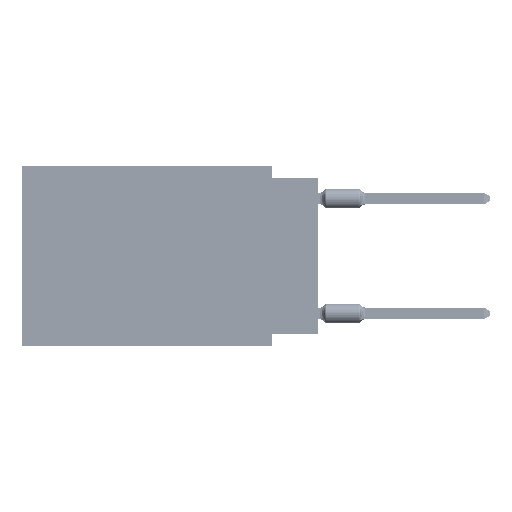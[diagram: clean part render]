
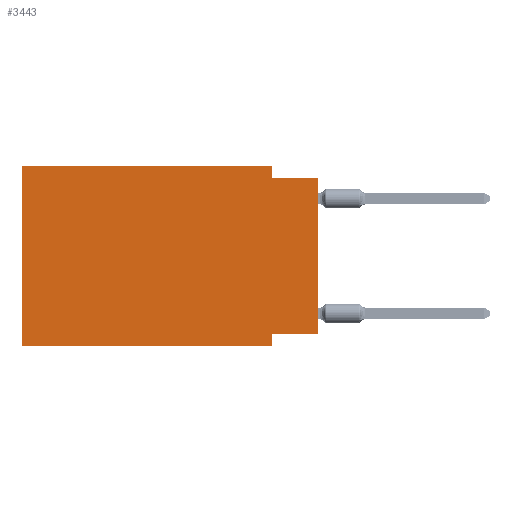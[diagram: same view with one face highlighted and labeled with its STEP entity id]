
A CAD part, left-side view. The second image highlights one B-rep face of the part: STEP entity #3443.
In plain terms, the highlighted planar face has unit normal (-1, 0, 0).
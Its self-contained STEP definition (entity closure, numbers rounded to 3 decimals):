
#3443 = ADVANCED_FACE ( 'NONE', ( #73398 ), #48200, .F. ) ;
#3777 = CARTESIAN_POINT ( 'NONE',  ( 0., 16.383, -9.906 ) ) ;
#6930 = VECTOR ( 'NONE', #9589, 1000. ) ;
#7085 = LINE ( 'NONE', #56255, #73986 ) ;
#7325 = LINE ( 'NONE', #38696, #23880 ) ;
#7594 = EDGE_CURVE ( 'NONE', #34533, #52376, #45774, .T. ) ;
#8217 = VERTEX_POINT ( 'NONE', #70680 ) ;
#9589 = DIRECTION ( 'NONE',  ( 0., -1., 0. ) ) ;
#9990 = LINE ( 'NONE', #3777, #6930 ) ;
#12648 = EDGE_LOOP ( 'NONE', ( #13565, #73922, #52273, #21023, #25241, #41100, #47008, #46604 ) ) ;
#13565 = ORIENTED_EDGE ( 'NONE', *, *, #61084, .T. ) ;
#16958 = EDGE_CURVE ( 'NONE', #50611, #20194, #9990, .T. ) ;
#19933 = DIRECTION ( 'NONE',  ( 0., 0., -1. ) ) ;
#20194 = VERTEX_POINT ( 'NONE', #63922 ) ;
#21023 = ORIENTED_EDGE ( 'NONE', *, *, #24905, .F. ) ;
#21789 = DIRECTION ( 'NONE',  ( 0., -1., 0. ) ) ;
#23021 = DIRECTION ( 'NONE',  ( 0., 0., -1. ) ) ;
#23880 = VECTOR ( 'NONE', #32113, 1000. ) ;
#24905 = EDGE_CURVE ( 'NONE', #73498, #34533, #7085, .T. ) ;
#25241 = ORIENTED_EDGE ( 'NONE', *, *, #78553, .F. ) ;
#26257 = VECTOR ( 'NONE', #19933, 1000. ) ;
#26548 = CARTESIAN_POINT ( 'NONE',  ( 0., 2.54, -9.906 ) ) ;
#28458 = CARTESIAN_POINT ( 'NONE',  ( 0., 16.383, 0. ) ) ;
#29220 = DIRECTION ( 'NONE',  ( 1., 0., 0. ) ) ;
#29319 = CARTESIAN_POINT ( 'NONE',  ( 0., 2.54, -9.271 ) ) ;
#29697 = CARTESIAN_POINT ( 'NONE',  ( 0., 2.54, -0.635 ) ) ;
#29850 = DIRECTION ( 'NONE',  ( 0., 1., 0. ) ) ;
#32113 = DIRECTION ( 'NONE',  ( 0., 0., 1. ) ) ;
#34517 = EDGE_CURVE ( 'NONE', #54607, #51164, #46826, .T. ) ;
#34533 = VERTEX_POINT ( 'NONE', #59631 ) ;
#36315 = VECTOR ( 'NONE', #80869, 1000. ) ;
#36653 = LINE ( 'NONE', #68861, #36315 ) ;
#37709 = LINE ( 'NONE', #26548, #26257 ) ;
#38696 = CARTESIAN_POINT ( 'NONE',  ( 0., 0., 0. ) ) ;
#39715 = AXIS2_PLACEMENT_3D ( 'NONE', #41190, #29220, #23021 ) ;
#41100 = ORIENTED_EDGE ( 'NONE', *, *, #16958, .T. ) ;
#41190 = CARTESIAN_POINT ( 'NONE',  ( 0., 16.383, 0. ) ) ;
#45774 = LINE ( 'NONE', #53606, #58546 ) ;
#46604 = ORIENTED_EDGE ( 'NONE', *, *, #34517, .F. ) ;
#46661 = CARTESIAN_POINT ( 'NONE',  ( 0., 0., -9.271 ) ) ;
#46826 = LINE ( 'NONE', #72015, #73651 ) ;
#47008 = ORIENTED_EDGE ( 'NONE', *, *, #67444, .F. ) ;
#48200 = PLANE ( 'NONE',  #39715 ) ;
#50611 = VERTEX_POINT ( 'NONE', #63854 ) ;
#50863 = DIRECTION ( 'NONE',  ( 0., -1., 0. ) ) ;
#51164 = VERTEX_POINT ( 'NONE', #29319 ) ;
#52273 = ORIENTED_EDGE ( 'NONE', *, *, #7594, .F. ) ;
#52376 = VERTEX_POINT ( 'NONE', #29697 ) ;
#53606 = CARTESIAN_POINT ( 'NONE',  ( 0., 2.54, 0. ) ) ;
#54607 = VERTEX_POINT ( 'NONE', #46661 ) ;
#56255 = CARTESIAN_POINT ( 'NONE',  ( 0., 16.383, 0. ) ) ;
#58546 = VECTOR ( 'NONE', #78404, 1000. ) ;
#58986 = CARTESIAN_POINT ( 'NONE',  ( 0., 0., -0.635 ) ) ;
#59631 = CARTESIAN_POINT ( 'NONE',  ( 0., 2.54, 0. ) ) ;
#61084 = EDGE_CURVE ( 'NONE', #54607, #8217, #7325, .T. ) ;
#63854 = CARTESIAN_POINT ( 'NONE',  ( 0., 16.383, -9.906 ) ) ;
#63922 = CARTESIAN_POINT ( 'NONE',  ( 0., 2.54, -9.906 ) ) ;
#67444 = EDGE_CURVE ( 'NONE', #51164, #20194, #37709, .T. ) ;
#68426 = EDGE_CURVE ( 'NONE', #52376, #8217, #78383, .T. ) ;
#68861 = CARTESIAN_POINT ( 'NONE',  ( 0., 16.383, 0. ) ) ;
#70680 = CARTESIAN_POINT ( 'NONE',  ( 0., 0., -0.635 ) ) ;
#72015 = CARTESIAN_POINT ( 'NONE',  ( 0., 0., -9.271 ) ) ;
#73398 = FACE_OUTER_BOUND ( 'NONE', #12648, .T. ) ;
#73498 = VERTEX_POINT ( 'NONE', #28458 ) ;
#73651 = VECTOR ( 'NONE', #29850, 1000. ) ;
#73922 = ORIENTED_EDGE ( 'NONE', *, *, #68426, .F. ) ;
#73986 = VECTOR ( 'NONE', #50863, 1000. ) ;
#76493 = VECTOR ( 'NONE', #21789, 1000. ) ;
#78383 = LINE ( 'NONE', #58986, #76493 ) ;
#78404 = DIRECTION ( 'NONE',  ( 0., 0., -1. ) ) ;
#78553 = EDGE_CURVE ( 'NONE', #50611, #73498, #36653, .T. ) ;
#80869 = DIRECTION ( 'NONE',  ( 0., 0., 1. ) ) ;
